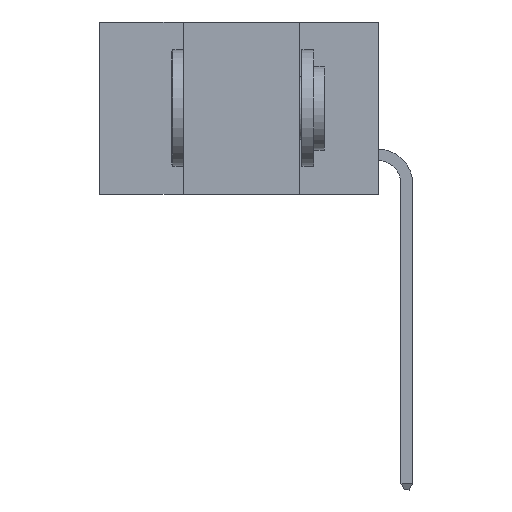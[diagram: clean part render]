
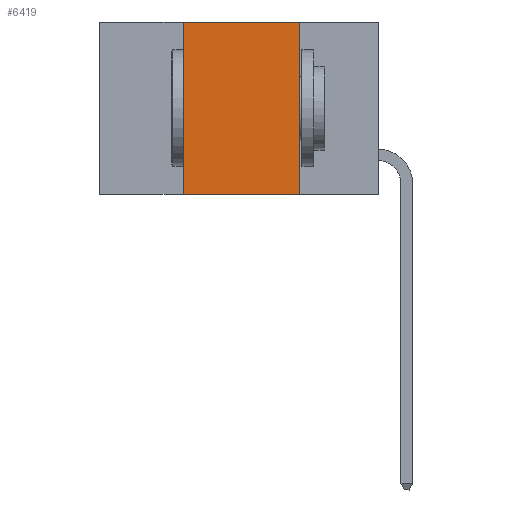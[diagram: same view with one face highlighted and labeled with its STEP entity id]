
A CAD part, left-side view. The second image highlights one B-rep face of the part: STEP entity #6419.
In plain terms, the highlighted planar face has unit normal (-1, 0, 0).
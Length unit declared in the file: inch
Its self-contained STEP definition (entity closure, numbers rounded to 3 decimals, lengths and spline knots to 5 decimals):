
#39 = VERTEX_POINT ( 'NONE', #9789 ) ;
#255 = EDGE_CURVE ( 'NONE', #39, #3755, #2266, .T. ) ;
#593 = CARTESIAN_POINT ( 'NONE',  ( 0., 0.42, 0. ) ) ;
#669 = DIRECTION ( 'NONE',  ( 0., 0., 1. ) ) ;
#848 = VERTEX_POINT ( 'NONE', #8947 ) ;
#2266 = LINE ( 'NONE', #593, #10725 ) ;
#2653 = ORIENTED_EDGE ( 'NONE', *, *, #7982, .F. ) ;
#3168 = VECTOR ( 'NONE', #3316, 39.37008 ) ;
#3316 = DIRECTION ( 'NONE',  ( 0., -1., 0. ) ) ;
#3511 = VERTEX_POINT ( 'NONE', #7848 ) ;
#3755 = VERTEX_POINT ( 'NONE', #6227 ) ;
#3954 = CARTESIAN_POINT ( 'NONE',  ( 0., 0.6, 0. ) ) ;
#5765 = VECTOR ( 'NONE', #7024, 39.37008 ) ;
#5822 = VECTOR ( 'NONE', #6090, 39.37008 ) ;
#5889 = EDGE_CURVE ( 'NONE', #3755, #848, #6014, .T. ) ;
#6014 = LINE ( 'NONE', #3954, #3168 ) ;
#6090 = DIRECTION ( 'NONE',  ( 0., -1., 0. ) ) ;
#6190 = CARTESIAN_POINT ( 'NONE',  ( 0., 0.17, 0. ) ) ;
#6227 = CARTESIAN_POINT ( 'NONE',  ( 0., 0.42, 0. ) ) ;
#6419 = ADVANCED_FACE ( 'NONE', ( #6672 ), #10911, .F. ) ;
#6672 = FACE_OUTER_BOUND ( 'NONE', #9348, .T. ) ;
#6815 = ORIENTED_EDGE ( 'NONE', *, *, #10793, .T. ) ;
#7024 = DIRECTION ( 'NONE',  ( 0., 0., -1. ) ) ;
#7848 = CARTESIAN_POINT ( 'NONE',  ( 0., 0.17, -0.37 ) ) ;
#7982 = EDGE_CURVE ( 'NONE', #848, #3511, #10174, .T. ) ;
#8562 = CARTESIAN_POINT ( 'NONE',  ( 0., 0.6, -0.37 ) ) ;
#8946 = DIRECTION ( 'NONE',  ( 0., 0., -1. ) ) ;
#8947 = CARTESIAN_POINT ( 'NONE',  ( 0., 0.17, 0. ) ) ;
#9116 = DIRECTION ( 'NONE',  ( 1., 0., 0. ) ) ;
#9348 = EDGE_LOOP ( 'NONE', ( #2653, #10024, #10621, #6815 ) ) ;
#9789 = CARTESIAN_POINT ( 'NONE',  ( 0., 0.42, -0.37 ) ) ;
#10024 = ORIENTED_EDGE ( 'NONE', *, *, #5889, .F. ) ;
#10174 = LINE ( 'NONE', #6190, #5765 ) ;
#10241 = LINE ( 'NONE', #8562, #5822 ) ;
#10621 = ORIENTED_EDGE ( 'NONE', *, *, #255, .F. ) ;
#10725 = VECTOR ( 'NONE', #669, 39.37008 ) ;
#10793 = EDGE_CURVE ( 'NONE', #39, #3511, #10241, .T. ) ;
#10800 = AXIS2_PLACEMENT_3D ( 'NONE', #10912, #9116, #8946 ) ;
#10911 = PLANE ( 'NONE',  #10800 ) ;
#10912 = CARTESIAN_POINT ( 'NONE',  ( 0., 0.6, 0. ) ) ;
